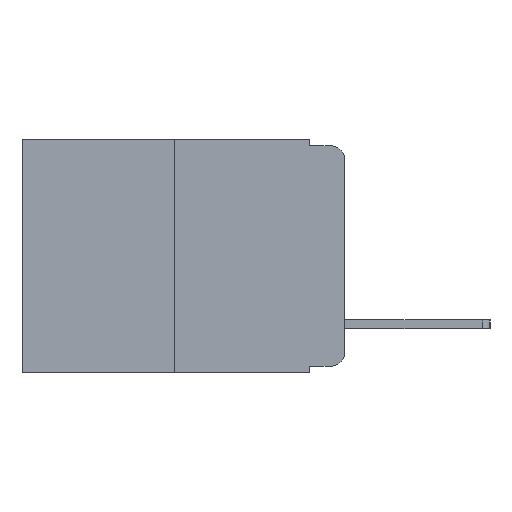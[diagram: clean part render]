
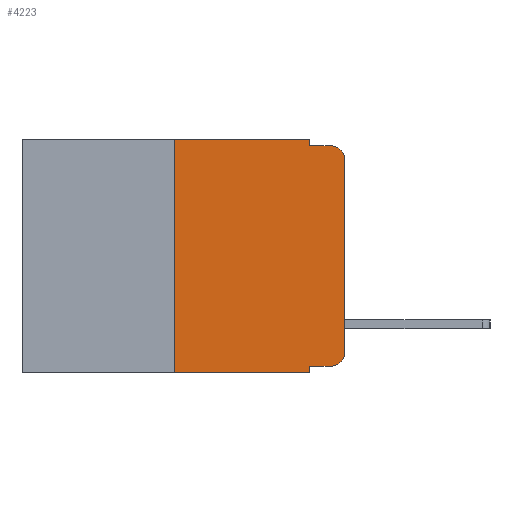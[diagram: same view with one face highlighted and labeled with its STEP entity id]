
A CAD part, left-side view. The second image highlights one B-rep face of the part: STEP entity #4223.
In plain terms, the highlighted planar face has unit normal (-1, 0, 0).
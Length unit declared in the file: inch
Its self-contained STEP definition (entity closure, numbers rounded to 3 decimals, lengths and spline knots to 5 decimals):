
#385 = ORIENTED_EDGE ( 'NONE', *, *, #15891, .F. ) ;
#578 = CARTESIAN_POINT ( 'NONE',  ( 0., 0.473, 0. ) ) ;
#847 = VECTOR ( 'NONE', #16934, 39.37008 ) ;
#923 = VERTEX_POINT ( 'NONE', #12534 ) ;
#1017 = EDGE_CURVE ( 'NONE', #15038, #14328, #10472, .T. ) ;
#1038 = EDGE_CURVE ( 'NONE', #1754, #9791, #13835, .T. ) ;
#1559 = EDGE_CURVE ( 'NONE', #5171, #2077, #12277, .T. ) ;
#1571 = CARTESIAN_POINT ( 'NONE',  ( 0., 0.02, -0.01 ) ) ;
#1691 = ORIENTED_EDGE ( 'NONE', *, *, #1038, .F. ) ;
#1754 = VERTEX_POINT ( 'NONE', #15867 ) ;
#2077 = VERTEX_POINT ( 'NONE', #17022 ) ;
#2078 = CARTESIAN_POINT ( 'NONE',  ( 0., 0.051, -0.01 ) ) ;
#2309 = ORIENTED_EDGE ( 'NONE', *, *, #17445, .F. ) ;
#2339 = VECTOR ( 'NONE', #11384, 39.37008 ) ;
#2349 = ORIENTED_EDGE ( 'NONE', *, *, #5410, .T. ) ;
#2393 = ORIENTED_EDGE ( 'NONE', *, *, #4882, .T. ) ;
#2459 = FACE_OUTER_BOUND ( 'NONE', #2625, .T. ) ;
#2625 = EDGE_LOOP ( 'NONE', ( #6815, #6257, #2728, #2309, #1691, #385, #2349, #3200, #2956, #2393 ) ) ;
#2728 = ORIENTED_EDGE ( 'NONE', *, *, #1017, .F. ) ;
#2821 = DIRECTION ( 'NONE',  ( 0., 0., -1. ) ) ;
#2956 = ORIENTED_EDGE ( 'NONE', *, *, #13170, .T. ) ;
#3200 = ORIENTED_EDGE ( 'NONE', *, *, #1559, .F. ) ;
#3379 = AXIS2_PLACEMENT_3D ( 'NONE', #16496, #7948, #17894 ) ;
#3690 = CARTESIAN_POINT ( 'NONE',  ( 0., 0., 0. ) ) ;
#3925 = VECTOR ( 'NONE', #5696, 39.37008 ) ;
#4223 = ADVANCED_FACE ( 'NONE', ( #2459 ), #18899, .F. ) ;
#4834 = CIRCLE ( 'NONE', #3379, 0.02 ) ;
#4882 = EDGE_CURVE ( 'NONE', #923, #17852, #4834, .T. ) ;
#5171 = VERTEX_POINT ( 'NONE', #17233 ) ;
#5227 = VERTEX_POINT ( 'NONE', #14640 ) ;
#5242 = CARTESIAN_POINT ( 'NONE',  ( 0., 0., -0.03 ) ) ;
#5410 = EDGE_CURVE ( 'NONE', #5227, #2077, #6011, .T. ) ;
#5467 = CARTESIAN_POINT ( 'NONE',  ( 0., 0.051, -0.01 ) ) ;
#5503 = VECTOR ( 'NONE', #10037, 39.37008 ) ;
#5613 = DIRECTION ( 'NONE',  ( 0., -1., 0. ) ) ;
#5696 = DIRECTION ( 'NONE',  ( 0., 0., 1. ) ) ;
#6011 = LINE ( 'NONE', #18034, #13303 ) ;
#6020 = VERTEX_POINT ( 'NONE', #5242 ) ;
#6257 = ORIENTED_EDGE ( 'NONE', *, *, #13871, .T. ) ;
#6572 = DIRECTION ( 'NONE',  ( 0., -1., 0. ) ) ;
#6815 = ORIENTED_EDGE ( 'NONE', *, *, #10556, .T. ) ;
#7081 = AXIS2_PLACEMENT_3D ( 'NONE', #10403, #11873, #2821 ) ;
#7948 = DIRECTION ( 'NONE',  ( -1., 0., 0. ) ) ;
#8439 = VECTOR ( 'NONE', #18615, 39.37008 ) ;
#8456 = DIRECTION ( 'NONE',  ( -1., 0., 0. ) ) ;
#8643 = CARTESIAN_POINT ( 'NONE',  ( 0., 0.25, 0. ) ) ;
#8661 = CARTESIAN_POINT ( 'NONE',  ( 0., 0.051, 0. ) ) ;
#9430 = LINE ( 'NONE', #14281, #5503 ) ;
#9791 = VERTEX_POINT ( 'NONE', #8661 ) ;
#10037 = DIRECTION ( 'NONE',  ( 0., -1., 0. ) ) ;
#10129 = LINE ( 'NONE', #3690, #847 ) ;
#10403 = CARTESIAN_POINT ( 'NONE',  ( 0., 0.473, 0. ) ) ;
#10472 = LINE ( 'NONE', #5467, #2339 ) ;
#10556 = EDGE_CURVE ( 'NONE', #17852, #6020, #10129, .T. ) ;
#10777 = CARTESIAN_POINT ( 'NONE',  ( 0., 0., -0.313 ) ) ;
#11384 = DIRECTION ( 'NONE',  ( 0., -1., 0. ) ) ;
#11568 = CARTESIAN_POINT ( 'NONE',  ( 0., 0.051, 0. ) ) ;
#11822 = VECTOR ( 'NONE', #12358, 39.37008 ) ;
#11873 = DIRECTION ( 'NONE',  ( 1., 0., 0. ) ) ;
#12277 = LINE ( 'NONE', #19346, #11822 ) ;
#12358 = DIRECTION ( 'NONE',  ( 0., 0., -1. ) ) ;
#12534 = CARTESIAN_POINT ( 'NONE',  ( 0., 0.02, -0.333 ) ) ;
#13170 = EDGE_CURVE ( 'NONE', #5171, #923, #9430, .T. ) ;
#13303 = VECTOR ( 'NONE', #6572, 39.37008 ) ;
#13403 = VECTOR ( 'NONE', #5613, 39.37008 ) ;
#13835 = LINE ( 'NONE', #578, #13403 ) ;
#13871 = EDGE_CURVE ( 'NONE', #6020, #14328, #15483, .T. ) ;
#14281 = CARTESIAN_POINT ( 'NONE',  ( 0., 0.051, -0.333 ) ) ;
#14328 = VERTEX_POINT ( 'NONE', #1571 ) ;
#14640 = CARTESIAN_POINT ( 'NONE',  ( 0., 0.25, -0.343 ) ) ;
#15038 = VERTEX_POINT ( 'NONE', #2078 ) ;
#15483 = CIRCLE ( 'NONE', #15629, 0.02 ) ;
#15629 = AXIS2_PLACEMENT_3D ( 'NONE', #16987, #8456, #18408 ) ;
#15867 = CARTESIAN_POINT ( 'NONE',  ( 0., 0.25, 0. ) ) ;
#15891 = EDGE_CURVE ( 'NONE', #5227, #1754, #19338, .T. ) ;
#16035 = LINE ( 'NONE', #11568, #8439 ) ;
#16496 = CARTESIAN_POINT ( 'NONE',  ( 0., 0.02, -0.313 ) ) ;
#16934 = DIRECTION ( 'NONE',  ( 0., 0., 1. ) ) ;
#16987 = CARTESIAN_POINT ( 'NONE',  ( 0., 0.02, -0.03 ) ) ;
#17022 = CARTESIAN_POINT ( 'NONE',  ( 0., 0.051, -0.343 ) ) ;
#17233 = CARTESIAN_POINT ( 'NONE',  ( 0., 0.051, -0.333 ) ) ;
#17445 = EDGE_CURVE ( 'NONE', #9791, #15038, #16035, .T. ) ;
#17852 = VERTEX_POINT ( 'NONE', #10777 ) ;
#17894 = DIRECTION ( 'NONE',  ( 0., 0., -1. ) ) ;
#18034 = CARTESIAN_POINT ( 'NONE',  ( 0., 0.473, -0.343 ) ) ;
#18408 = DIRECTION ( 'NONE',  ( 0., 0., -1. ) ) ;
#18615 = DIRECTION ( 'NONE',  ( 0., 0., -1. ) ) ;
#18899 = PLANE ( 'NONE',  #7081 ) ;
#19338 = LINE ( 'NONE', #8643, #3925 ) ;
#19346 = CARTESIAN_POINT ( 'NONE',  ( 0., 0.051, 0. ) ) ;
